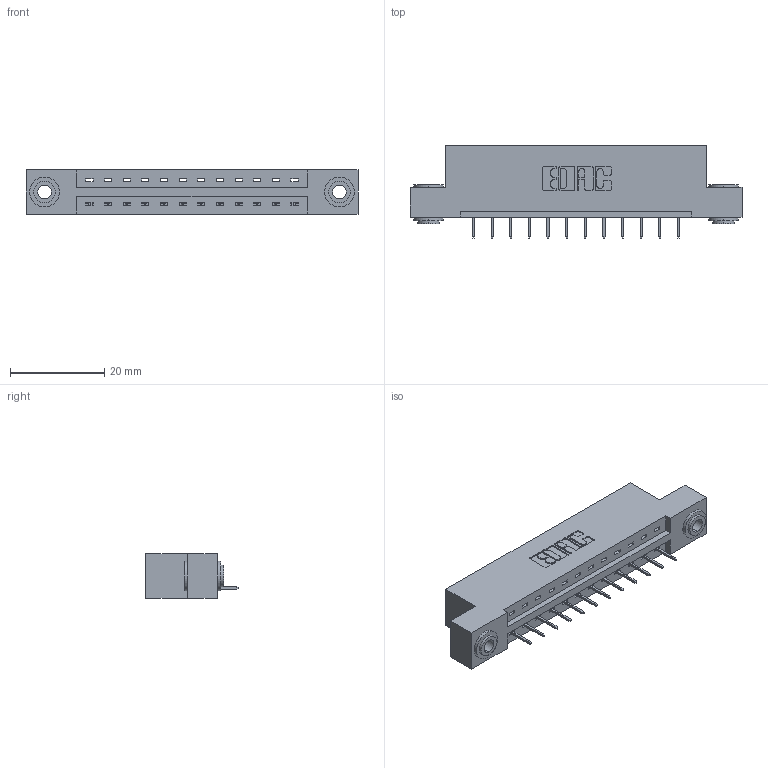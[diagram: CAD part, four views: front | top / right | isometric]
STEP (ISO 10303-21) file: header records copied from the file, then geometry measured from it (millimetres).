
FILE_DESCRIPTION (( 'STEP AP203' ), '1' );
FILE_NAME ('387-012-524-103.STEP', '2019-10-02T13:07:16', ( '' ), ( '' ), 'SwSTEP 2.0', 'SolidWorks 2016', '' );
FILE_SCHEMA (( 'CONFIG_CONTROL_DESIGN' ));
Length unit declared in the file: inch
Products named in the file (4): 345-250-002_345-250-002-102; 337 Part_Flush Mounting Lugs - 0.156 Dia-TH; 387-012-524-103; 345-292-001_345-293-124
Assembly tree (15 placements, depth 2):
  387-012-524-103
    337 Part_Flush Mounting Lugs - 0.156 Dia-TH
    345-292-001_345-293-124  x12
    345-250-002_345-250-002-102  x2
Bounding box: 70.56 x 19.69 x 9.4 mm (x, y, z)
Volume: 6930.2 mm3; surface area: 7060.9 mm2
Topology: 15 solids, 15 shells, 944 faces, 2691 edges, 1742 vertices
Faces by surface type: plane 704, cylinder 232, cone 8
Entity records: 13524 total; most frequent: CARTESIAN_POINT 2329, ORIENTED_EDGE 2270, DIRECTION 2057, EDGE_CURVE 1135, LINE 987, VECTOR 987, VERTEX_POINT 750, AXIS2_PLACEMENT_3D 535
